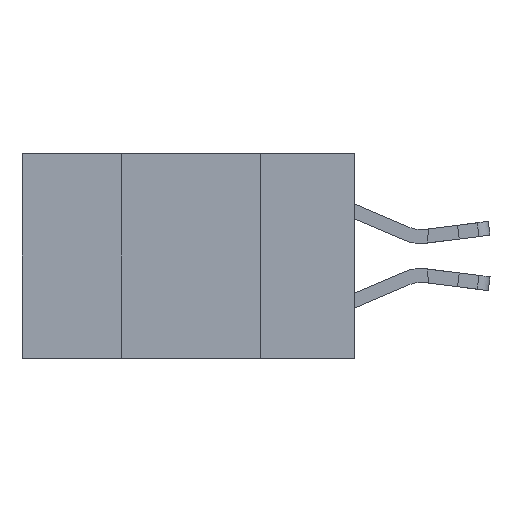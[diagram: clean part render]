
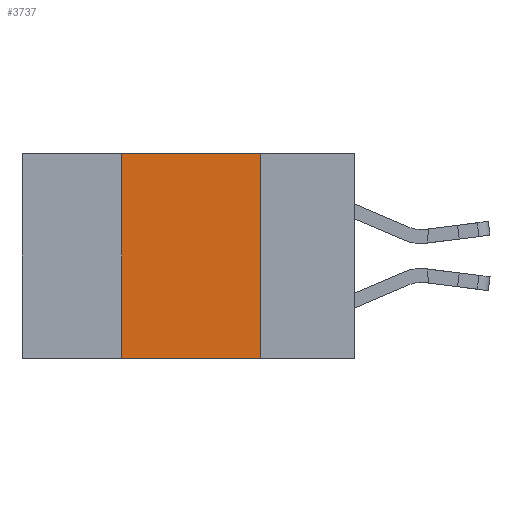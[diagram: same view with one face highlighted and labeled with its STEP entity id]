
A CAD part, left-side view. The second image highlights one B-rep face of the part: STEP entity #3737.
In plain terms, the highlighted planar face has unit normal (-1, 0, 0).
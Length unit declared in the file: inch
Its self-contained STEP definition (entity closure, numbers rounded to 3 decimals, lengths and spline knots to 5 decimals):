
#187 = EDGE_CURVE ( 'NONE', #10411, #5160, #8890, .T. ) ;
#487 = EDGE_CURVE ( 'NONE', #6694, #645, #6795, .T. ) ;
#572 = VECTOR ( 'NONE', #745, 39.37008 ) ;
#645 = VERTEX_POINT ( 'NONE', #5352 ) ;
#745 = DIRECTION ( 'NONE',  ( 0., -1., 0. ) ) ;
#921 = VECTOR ( 'NONE', #2332, 39.37008 ) ;
#1282 = VECTOR ( 'NONE', #14098, 39.37008 ) ;
#2073 = EDGE_LOOP ( 'NONE', ( #3899, #2598, #12769, #9823 ) ) ;
#2238 = DIRECTION ( 'NONE',  ( 0., 0., 1. ) ) ;
#2325 = CARTESIAN_POINT ( 'NONE',  ( 0., 0.42, 0. ) ) ;
#2332 = DIRECTION ( 'NONE',  ( 0., -1., 0. ) ) ;
#2598 = ORIENTED_EDGE ( 'NONE', *, *, #487, .F. ) ;
#2677 = CARTESIAN_POINT ( 'NONE',  ( 0., 0.42, -0.37 ) ) ;
#3737 = ADVANCED_FACE ( 'NONE', ( #4098 ), #9700, .F. ) ;
#3899 = ORIENTED_EDGE ( 'NONE', *, *, #13703, .F. ) ;
#4093 = DIRECTION ( 'NONE',  ( 0., 0., -1. ) ) ;
#4098 = FACE_OUTER_BOUND ( 'NONE', #2073, .T. ) ;
#4198 = DIRECTION ( 'NONE',  ( 1., 0., 0. ) ) ;
#4223 = LINE ( 'NONE', #13088, #1282 ) ;
#4402 = CARTESIAN_POINT ( 'NONE',  ( 0., 0.42, 0. ) ) ;
#5160 = VERTEX_POINT ( 'NONE', #12717 ) ;
#5352 = CARTESIAN_POINT ( 'NONE',  ( 0., 0.17, 0. ) ) ;
#6219 = CARTESIAN_POINT ( 'NONE',  ( 0., 0.6, 0. ) ) ;
#6694 = VERTEX_POINT ( 'NONE', #4402 ) ;
#6795 = LINE ( 'NONE', #6219, #572 ) ;
#6839 = VECTOR ( 'NONE', #2238, 39.37008 ) ;
#8890 = LINE ( 'NONE', #9954, #921 ) ;
#9108 = EDGE_CURVE ( 'NONE', #10411, #6694, #9795, .T. ) ;
#9700 = PLANE ( 'NONE',  #12045 ) ;
#9795 = LINE ( 'NONE', #2325, #6839 ) ;
#9823 = ORIENTED_EDGE ( 'NONE', *, *, #187, .T. ) ;
#9954 = CARTESIAN_POINT ( 'NONE',  ( 0., 0.6, -0.37 ) ) ;
#10411 = VERTEX_POINT ( 'NONE', #2677 ) ;
#12045 = AXIS2_PLACEMENT_3D ( 'NONE', #12955, #4198, #4093 ) ;
#12717 = CARTESIAN_POINT ( 'NONE',  ( 0., 0.17, -0.37 ) ) ;
#12769 = ORIENTED_EDGE ( 'NONE', *, *, #9108, .F. ) ;
#12955 = CARTESIAN_POINT ( 'NONE',  ( 0., 0.6, 0. ) ) ;
#13088 = CARTESIAN_POINT ( 'NONE',  ( 0., 0.17, 0. ) ) ;
#13703 = EDGE_CURVE ( 'NONE', #645, #5160, #4223, .T. ) ;
#14098 = DIRECTION ( 'NONE',  ( 0., 0., -1. ) ) ;
